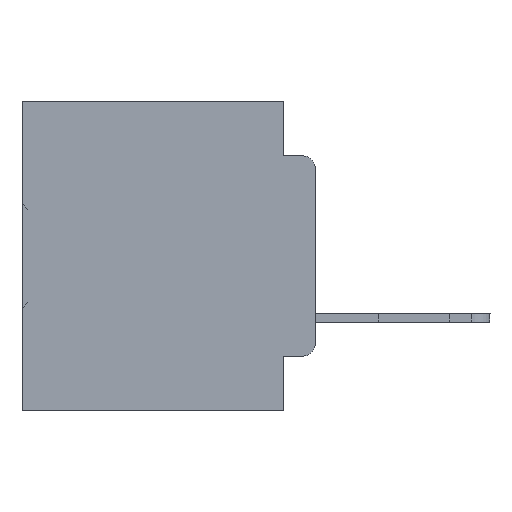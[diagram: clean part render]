
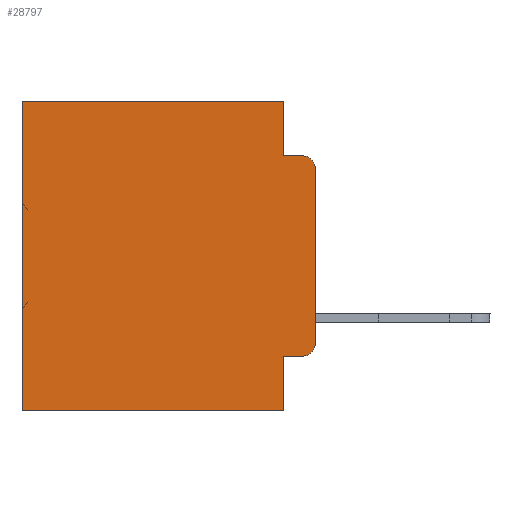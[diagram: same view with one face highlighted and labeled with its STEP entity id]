
A CAD part, left-side view. The second image highlights one B-rep face of the part: STEP entity #28797.
In plain terms, the highlighted planar face has unit normal (-1, 0, 0).
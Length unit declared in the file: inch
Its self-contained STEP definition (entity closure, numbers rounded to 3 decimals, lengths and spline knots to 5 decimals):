
#391 = CARTESIAN_POINT ( 'NONE',  ( 0.298, 0.051, -0.4115 ) ) ;
#491 = VECTOR ( 'NONE', #10300, 39.37008 ) ;
#885 = VERTEX_POINT ( 'NONE', #5029 ) ;
#1473 = FACE_OUTER_BOUND ( 'NONE', #7676, .T. ) ;
#1736 = ORIENTED_EDGE ( 'NONE', *, *, #15125, .F. ) ;
#1991 = CARTESIAN_POINT ( 'NONE',  ( 0.298, 0.473, -0.5 ) ) ;
#2089 = VERTEX_POINT ( 'NONE', #19515 ) ;
#3425 = CARTESIAN_POINT ( 'NONE',  ( 0.298, 0.02, -0.1085 ) ) ;
#3757 = CARTESIAN_POINT ( 'NONE',  ( 0.298, 0.051, 0. ) ) ;
#4478 = VECTOR ( 'NONE', #17618, 39.37008 ) ;
#4649 = DIRECTION ( 'NONE',  ( 0., 0., -1. ) ) ;
#4721 = CARTESIAN_POINT ( 'NONE',  ( 0.298, 0.473, 0. ) ) ;
#5029 = CARTESIAN_POINT ( 'NONE',  ( 0.298, 0.051, -0.5 ) ) ;
#6007 = VECTOR ( 'NONE', #13121, 39.37008 ) ;
#6675 = VERTEX_POINT ( 'NONE', #19247 ) ;
#6875 = VERTEX_POINT ( 'NONE', #12375 ) ;
#7143 = DIRECTION ( 'NONE',  ( 0., 0., -1. ) ) ;
#7250 = CARTESIAN_POINT ( 'NONE',  ( 0.298, 0., 0. ) ) ;
#7320 = VERTEX_POINT ( 'NONE', #1991 ) ;
#7488 = VERTEX_POINT ( 'NONE', #22500 ) ;
#7490 = VECTOR ( 'NONE', #10129, 39.37008 ) ;
#7640 = PLANE ( 'NONE',  #9703 ) ;
#7676 = EDGE_LOOP ( 'NONE', ( #15445, #27176, #20238, #35788, #31228, #26433, #13980, #1736, #26444, #35425 ) ) ;
#8209 = EDGE_CURVE ( 'NONE', #6875, #7488, #24239, .T. ) ;
#8475 = DIRECTION ( 'NONE',  ( 0., 1., 0. ) ) ;
#9703 = AXIS2_PLACEMENT_3D ( 'NONE', #21980, #19141, #16308 ) ;
#10129 = DIRECTION ( 'NONE',  ( 0., 0., -1. ) ) ;
#10300 = DIRECTION ( 'NONE',  ( 0., 0., -1. ) ) ;
#10743 = EDGE_CURVE ( 'NONE', #14994, #6675, #22987, .T. ) ;
#11813 = AXIS2_PLACEMENT_3D ( 'NONE', #17502, #14664, #28975 ) ;
#11829 = EDGE_CURVE ( 'NONE', #885, #7320, #24002, .T. ) ;
#11870 = DIRECTION ( 'NONE',  ( 0., 0., -1. ) ) ;
#12375 = CARTESIAN_POINT ( 'NONE',  ( 0.298, 0.051, -0.0885 ) ) ;
#12589 = VERTEX_POINT ( 'NONE', #391 ) ;
#12943 = LINE ( 'NONE', #35921, #7490 ) ;
#13121 = DIRECTION ( 'NONE',  ( 0., -1., 0. ) ) ;
#13980 = ORIENTED_EDGE ( 'NONE', *, *, #11829, .F. ) ;
#14311 = CARTESIAN_POINT ( 'NONE',  ( 0.298, 0.051, 0. ) ) ;
#14447 = CARTESIAN_POINT ( 'NONE',  ( 0.298, 0.02, -0.4115 ) ) ;
#14664 = DIRECTION ( 'NONE',  ( -1., 0., 0. ) ) ;
#14884 = VECTOR ( 'NONE', #32242, 39.37008 ) ;
#14885 = DIRECTION ( 'NONE',  ( -1., 0., 0. ) ) ;
#14994 = VERTEX_POINT ( 'NONE', #14311 ) ;
#15125 = EDGE_CURVE ( 'NONE', #12589, #885, #24063, .T. ) ;
#15445 = ORIENTED_EDGE ( 'NONE', *, *, #32158, .F. ) ;
#16102 = LINE ( 'NONE', #7250, #35014 ) ;
#16308 = DIRECTION ( 'NONE',  ( 0., 0., -1. ) ) ;
#17502 = CARTESIAN_POINT ( 'NONE',  ( 0.298, 0.02, -0.3915 ) ) ;
#17618 = DIRECTION ( 'NONE',  ( 0., 1., 0. ) ) ;
#18995 = LINE ( 'NONE', #4721, #36196 ) ;
#19141 = DIRECTION ( 'NONE',  ( 1., 0., 0. ) ) ;
#19247 = CARTESIAN_POINT ( 'NONE',  ( 0.298, 0.473, 0. ) ) ;
#19515 = CARTESIAN_POINT ( 'NONE',  ( 0.298, 0., -0.1085 ) ) ;
#20238 = ORIENTED_EDGE ( 'NONE', *, *, #8209, .F. ) ;
#20786 = LINE ( 'NONE', #35066, #14884 ) ;
#21067 = EDGE_CURVE ( 'NONE', #35041, #23955, #33473, .T. ) ;
#21866 = VECTOR ( 'NONE', #8475, 39.37008 ) ;
#21980 = CARTESIAN_POINT ( 'NONE',  ( 0.298, 0., 0. ) ) ;
#22500 = CARTESIAN_POINT ( 'NONE',  ( 0.298, 0.02, -0.0885 ) ) ;
#22622 = CARTESIAN_POINT ( 'NONE',  ( 0.298, 0., 0. ) ) ;
#22987 = LINE ( 'NONE', #22622, #21866 ) ;
#23326 = EDGE_CURVE ( 'NONE', #12589, #35041, #20786, .T. ) ;
#23955 = VERTEX_POINT ( 'NONE', #27486 ) ;
#24002 = LINE ( 'NONE', #32103, #4478 ) ;
#24063 = LINE ( 'NONE', #3757, #491 ) ;
#24239 = LINE ( 'NONE', #33833, #6007 ) ;
#26433 = ORIENTED_EDGE ( 'NONE', *, *, #29672, .T. ) ;
#26444 = ORIENTED_EDGE ( 'NONE', *, *, #23326, .T. ) ;
#27176 = ORIENTED_EDGE ( 'NONE', *, *, #34658, .T. ) ;
#27486 = CARTESIAN_POINT ( 'NONE',  ( 0.298, 0., -0.3915 ) ) ;
#28797 = ADVANCED_FACE ( 'NONE', ( #1473 ), #7640, .F. ) ;
#28975 = DIRECTION ( 'NONE',  ( 0., 0., -1. ) ) ;
#29672 = EDGE_CURVE ( 'NONE', #6675, #7320, #18995, .T. ) ;
#31228 = ORIENTED_EDGE ( 'NONE', *, *, #10743, .T. ) ;
#32103 = CARTESIAN_POINT ( 'NONE',  ( 0.298, 0., -0.5 ) ) ;
#32158 = EDGE_CURVE ( 'NONE', #2089, #23955, #16102, .T. ) ;
#32242 = DIRECTION ( 'NONE',  ( 0., -1., 0. ) ) ;
#33473 = CIRCLE ( 'NONE', #11813, 0.02 ) ;
#33833 = CARTESIAN_POINT ( 'NONE',  ( 0.298, 0.051, -0.0885 ) ) ;
#33917 = AXIS2_PLACEMENT_3D ( 'NONE', #3425, #14885, #11870 ) ;
#34658 = EDGE_CURVE ( 'NONE', #2089, #7488, #35691, .T. ) ;
#35014 = VECTOR ( 'NONE', #4649, 39.37008 ) ;
#35041 = VERTEX_POINT ( 'NONE', #14447 ) ;
#35066 = CARTESIAN_POINT ( 'NONE',  ( 0.298, 0.051, -0.4115 ) ) ;
#35425 = ORIENTED_EDGE ( 'NONE', *, *, #21067, .T. ) ;
#35691 = CIRCLE ( 'NONE', #33917, 0.02 ) ;
#35788 = ORIENTED_EDGE ( 'NONE', *, *, #36239, .F. ) ;
#35921 = CARTESIAN_POINT ( 'NONE',  ( 0.298, 0.051, 0. ) ) ;
#36196 = VECTOR ( 'NONE', #7143, 39.37008 ) ;
#36239 = EDGE_CURVE ( 'NONE', #14994, #6875, #12943, .T. ) ;
